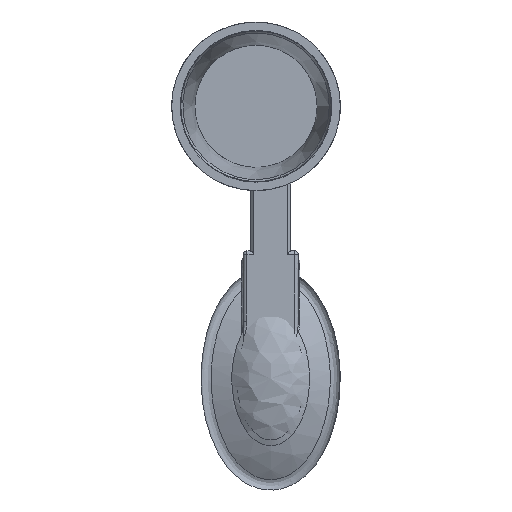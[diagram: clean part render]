
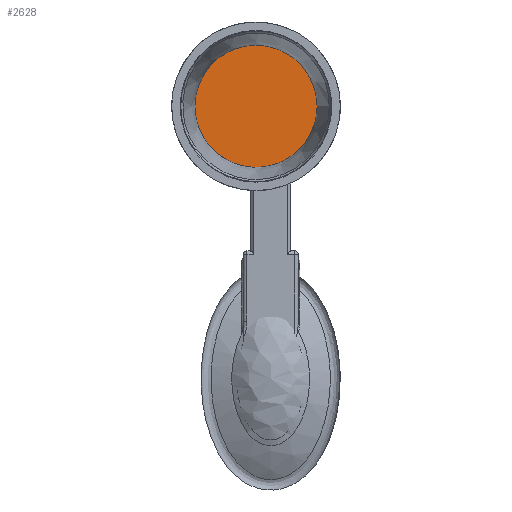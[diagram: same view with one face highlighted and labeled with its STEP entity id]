
A CAD part, left-side view. The second image highlights one B-rep face of the part: STEP entity #2628.
In plain terms, the highlighted planar face has unit normal (-1, 0, 0).
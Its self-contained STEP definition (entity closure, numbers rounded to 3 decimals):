
#338 = CARTESIAN_POINT ( 'NONE',  ( 86.318, 47.2, 8.3 ) ) ;
#992 = DIRECTION ( 'NONE',  ( 1., 0., 0. ) ) ;
#1207 = DIRECTION ( 'NONE',  ( 0., 0., -1. ) ) ;
#1772 = VERTEX_POINT ( 'NONE', #338 ) ;
#1898 = EDGE_LOOP ( 'NONE', ( #3056 ) ) ;
#2469 = CARTESIAN_POINT ( 'NONE',  ( 86.318, 47.2, 0. ) ) ;
#2539 = FACE_OUTER_BOUND ( 'NONE', #1898, .T. ) ;
#2628 = ADVANCED_FACE ( 'NONE', ( #2539 ), #4242, .T. ) ;
#2775 = AXIS2_PLACEMENT_3D ( 'NONE', #4220, #4262, #1207 ) ;
#2927 = AXIS2_PLACEMENT_3D ( 'NONE', #2469, #992, #3248 ) ;
#3056 = ORIENTED_EDGE ( 'NONE', *, *, #4376, .F. ) ;
#3248 = DIRECTION ( 'NONE',  ( 0., 0., 1. ) ) ;
#3683 = CIRCLE ( 'NONE', #2927, 8.3 ) ;
#4220 = CARTESIAN_POINT ( 'NONE',  ( 86.318, 55.501, 8.301 ) ) ;
#4242 = PLANE ( 'NONE',  #2775 ) ;
#4262 = DIRECTION ( 'NONE',  ( -1., 0., 0. ) ) ;
#4376 = EDGE_CURVE ( 'NONE', #1772, #1772, #3683, .T. ) ;
